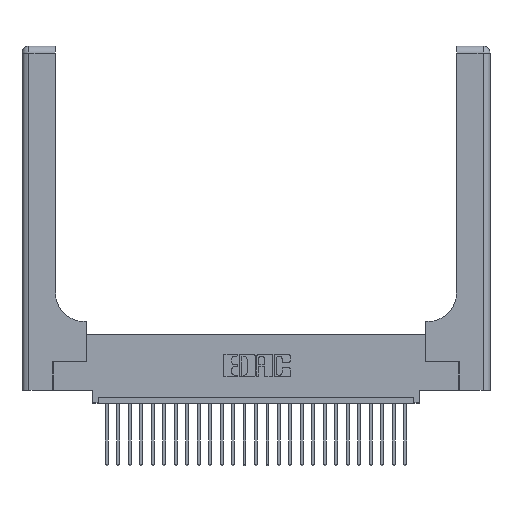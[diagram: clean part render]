
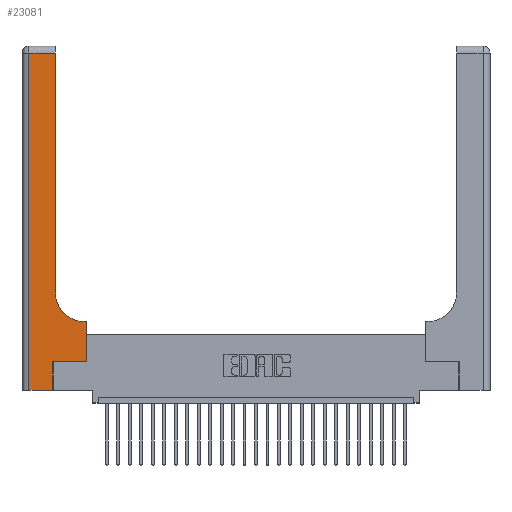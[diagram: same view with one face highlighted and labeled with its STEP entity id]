
A CAD part, top view. The second image highlights one B-rep face of the part: STEP entity #23081.
In plain terms, the highlighted planar face has unit normal (0, 0, 1).
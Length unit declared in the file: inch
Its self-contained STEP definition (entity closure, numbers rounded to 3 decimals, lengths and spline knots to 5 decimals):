
#300 = DIRECTION ( 'NONE',  ( -1., 0., 0. ) ) ;
#547 = ORIENTED_EDGE ( 'NONE', *, *, #18339, .T. ) ;
#1232 = VERTEX_POINT ( 'NONE', #10330 ) ;
#1292 = CARTESIAN_POINT ( 'NONE',  ( 0.269, 0.25, 0.37 ) ) ;
#1806 = ORIENTED_EDGE ( 'NONE', *, *, #27545, .T. ) ;
#3748 = LINE ( 'NONE', #4363, #16708 ) ;
#4284 = CIRCLE ( 'NONE', #19814, 0.25 ) ;
#4363 = CARTESIAN_POINT ( 'NONE',  ( 0.269, 0., 0.37 ) ) ;
#4591 = DIRECTION ( 'NONE',  ( 1., 0., 0. ) ) ;
#6220 = DIRECTION ( 'NONE',  ( -1., 0., 0. ) ) ;
#6346 = AXIS2_PLACEMENT_3D ( 'NONE', #19270, #6506, #6220 ) ;
#6506 = DIRECTION ( 'NONE',  ( 0., 0., -1. ) ) ;
#6902 = CARTESIAN_POINT ( 'NONE',  ( 0.2915, 0.85, 0.37 ) ) ;
#7179 = VECTOR ( 'NONE', #14844, 39.37008 ) ;
#7351 = VECTOR ( 'NONE', #4591, 39.37008 ) ;
#7892 = ORIENTED_EDGE ( 'NONE', *, *, #11922, .T. ) ;
#8137 = DIRECTION ( 'NONE',  ( 0., 0., -1. ) ) ;
#8351 = EDGE_CURVE ( 'NONE', #10435, #25149, #22946, .T. ) ;
#8537 = ORIENTED_EDGE ( 'NONE', *, *, #16886, .T. ) ;
#8616 = DIRECTION ( 'NONE',  ( 0., 1., 0. ) ) ;
#8842 = FACE_OUTER_BOUND ( 'NONE', #17728, .T. ) ;
#8958 = EDGE_CURVE ( 'NONE', #23385, #10989, #15833, .T. ) ;
#9105 = VECTOR ( 'NONE', #300, 39.37008 ) ;
#9267 = DIRECTION ( 'NONE',  ( 0., -1., 0. ) ) ;
#10254 = CARTESIAN_POINT ( 'NONE',  ( 0.5585, 0.6, 0.37 ) ) ;
#10330 = CARTESIAN_POINT ( 'NONE',  ( 0.06, 0., 0.37 ) ) ;
#10435 = VERTEX_POINT ( 'NONE', #13423 ) ;
#10445 = CARTESIAN_POINT ( 'NONE',  ( 0.2915, 0.6, 0.37 ) ) ;
#10932 = VECTOR ( 'NONE', #9267, 39.37008 ) ;
#10989 = VERTEX_POINT ( 'NONE', #25520 ) ;
#11319 = DIRECTION ( 'NONE',  ( -1., 0., 0. ) ) ;
#11922 = EDGE_CURVE ( 'NONE', #16254, #10435, #15985, .T. ) ;
#13043 = VERTEX_POINT ( 'NONE', #25239 ) ;
#13338 = CARTESIAN_POINT ( 'NONE',  ( 0., 2.94, 0.37 ) ) ;
#13423 = CARTESIAN_POINT ( 'NONE',  ( 0.5585, 0.25, 0.37 ) ) ;
#13444 = LINE ( 'NONE', #18980, #7179 ) ;
#14345 = ORIENTED_EDGE ( 'NONE', *, *, #25266, .T. ) ;
#14552 = LINE ( 'NONE', #21633, #17952 ) ;
#14844 = DIRECTION ( 'NONE',  ( 1., 0., 0. ) ) ;
#15241 = LINE ( 'NONE', #15397, #10932 ) ;
#15397 = CARTESIAN_POINT ( 'NONE',  ( 0.06, 3., 0.37 ) ) ;
#15589 = DIRECTION ( 'NONE',  ( 0., 1., 0. ) ) ;
#15833 = LINE ( 'NONE', #13338, #20885 ) ;
#15985 = LINE ( 'NONE', #17340, #7351 ) ;
#16254 = VERTEX_POINT ( 'NONE', #1292 ) ;
#16507 = CARTESIAN_POINT ( 'NONE',  ( 0.5415, 0.85, 0.37 ) ) ;
#16547 = EDGE_CURVE ( 'NONE', #10989, #1232, #15241, .T. ) ;
#16708 = VECTOR ( 'NONE', #8616, 39.37008 ) ;
#16886 = EDGE_CURVE ( 'NONE', #22832, #25526, #4284, .T. ) ;
#17340 = CARTESIAN_POINT ( 'NONE',  ( 0.269, 0.25, 0.37 ) ) ;
#17581 = VECTOR ( 'NONE', #15589, 39.37008 ) ;
#17722 = ORIENTED_EDGE ( 'NONE', *, *, #8351, .T. ) ;
#17728 = EDGE_LOOP ( 'NONE', ( #22077, #27591, #21490, #547, #1806, #7892, #17722, #14345, #8537 ) ) ;
#17952 = VECTOR ( 'NONE', #23629, 39.37008 ) ;
#18339 = EDGE_CURVE ( 'NONE', #1232, #13043, #13444, .T. ) ;
#18980 = CARTESIAN_POINT ( 'NONE',  ( 0., 0., 0.37 ) ) ;
#19270 = CARTESIAN_POINT ( 'NONE',  ( 0., 3., 0.37 ) ) ;
#19814 = AXIS2_PLACEMENT_3D ( 'NONE', #16507, #8137, #20740 ) ;
#20406 = CARTESIAN_POINT ( 'NONE',  ( 0.5415, 0.6, 0.37 ) ) ;
#20740 = DIRECTION ( 'NONE',  ( 1., 0., 0. ) ) ;
#20885 = VECTOR ( 'NONE', #11319, 39.37008 ) ;
#21490 = ORIENTED_EDGE ( 'NONE', *, *, #16547, .T. ) ;
#21608 = EDGE_CURVE ( 'NONE', #25526, #23385, #14552, .T. ) ;
#21633 = CARTESIAN_POINT ( 'NONE',  ( 0.2915, 3., 0.37 ) ) ;
#22077 = ORIENTED_EDGE ( 'NONE', *, *, #21608, .T. ) ;
#22168 = CARTESIAN_POINT ( 'NONE',  ( 0.2915, 2.94, 0.37 ) ) ;
#22832 = VERTEX_POINT ( 'NONE', #20406 ) ;
#22946 = LINE ( 'NONE', #26374, #17581 ) ;
#23081 = ADVANCED_FACE ( 'NONE', ( #8842 ), #27561, .F. ) ;
#23174 = LINE ( 'NONE', #10445, #9105 ) ;
#23385 = VERTEX_POINT ( 'NONE', #22168 ) ;
#23629 = DIRECTION ( 'NONE',  ( 0., 1., 0. ) ) ;
#25149 = VERTEX_POINT ( 'NONE', #10254 ) ;
#25239 = CARTESIAN_POINT ( 'NONE',  ( 0.269, 0., 0.37 ) ) ;
#25266 = EDGE_CURVE ( 'NONE', #25149, #22832, #23174, .T. ) ;
#25520 = CARTESIAN_POINT ( 'NONE',  ( 0.06, 2.94, 0.37 ) ) ;
#25526 = VERTEX_POINT ( 'NONE', #6902 ) ;
#26374 = CARTESIAN_POINT ( 'NONE',  ( 0.5585, 0.25, 0.37 ) ) ;
#27545 = EDGE_CURVE ( 'NONE', #13043, #16254, #3748, .T. ) ;
#27561 = PLANE ( 'NONE',  #6346 ) ;
#27591 = ORIENTED_EDGE ( 'NONE', *, *, #8958, .T. ) ;
